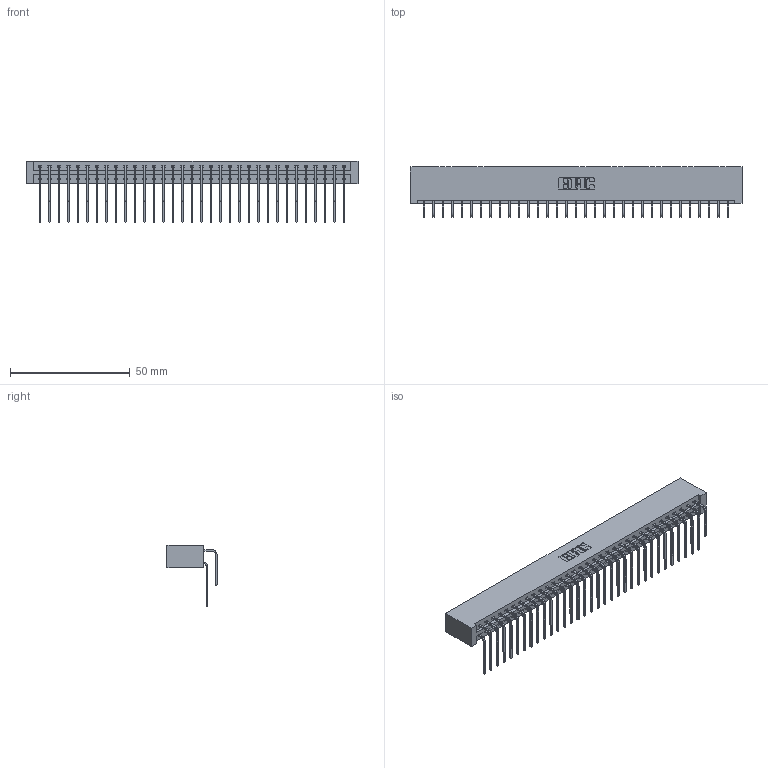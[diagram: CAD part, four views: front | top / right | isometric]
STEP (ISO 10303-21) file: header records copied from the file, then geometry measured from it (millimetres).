
FILE_DESCRIPTION (( 'STEP AP203' ), '1' );
FILE_NAME ('387-066-559-201.STEP', '2018-09-21T11:43:48', ( '' ), ( '' ), 'SwSTEP 2.0', 'SolidWorks 2016', '' );
FILE_SCHEMA (( 'CONFIG_CONTROL_DESIGN' ));
Length unit declared in the file: inch
Products named in the file (4): 387-066-559-201; 337 Part_No Mounting Lugs; 345-292-001_558 559 Tail - 1; 345-292-001_559 Tail - 2
Assembly tree (67 placements, depth 2):
  387-066-559-201
    337 Part_No Mounting Lugs
    345-292-001_558 559 Tail - 1  x33
    345-292-001_559 Tail - 2  x33
Bounding box: 138.63 x 20.9 x 25.53 mm (x, y, z)
Volume: 15631.9 mm3; surface area: 19552.4 mm2
Topology: 67 solids, 67 shells, 3802 faces, 11309 edges, 7450 vertices
Faces by surface type: plane 2706, cylinder 1096
Entity records: 28257 total; most frequent: CARTESIAN_POINT 4813, ORIENTED_EDGE 4698, DIRECTION 4085, EDGE_CURVE 2349, LINE 2189, VECTOR 2189, VERTEX_POINT 1562, AXIS2_PLACEMENT_3D 948
